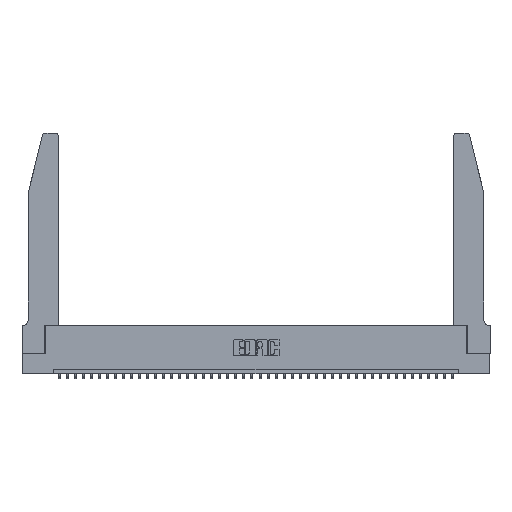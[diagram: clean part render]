
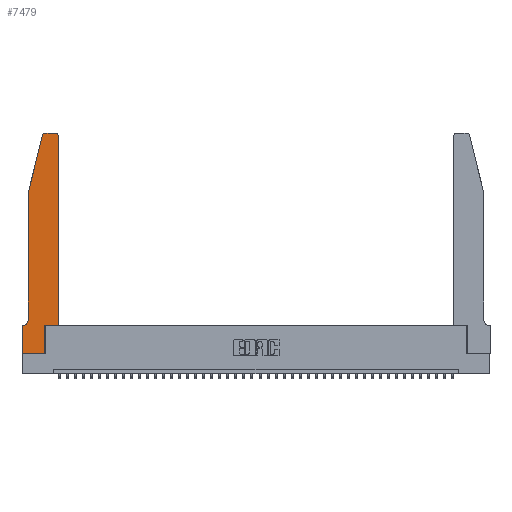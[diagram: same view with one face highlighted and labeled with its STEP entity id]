
A CAD part, top view. The second image highlights one B-rep face of the part: STEP entity #7479.
In plain terms, the highlighted planar face has unit normal (0, 0, 1).
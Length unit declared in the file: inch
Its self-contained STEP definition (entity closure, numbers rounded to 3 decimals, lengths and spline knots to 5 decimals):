
#445 = CIRCLE ( 'NONE', #5407, 0.07 ) ;
#660 = ORIENTED_EDGE ( 'NONE', *, *, #36651, .T. ) ;
#980 = LINE ( 'NONE', #1100, #13918 ) ;
#1089 = DIRECTION ( 'NONE',  ( 0., 1., 0. ) ) ;
#1100 = CARTESIAN_POINT ( 'NONE',  ( 0.0755, 0.35, 0.37 ) ) ;
#1144 = LINE ( 'NONE', #20333, #39673 ) ;
#2079 = VERTEX_POINT ( 'NONE', #34887 ) ;
#2639 = CARTESIAN_POINT ( 'NONE',  ( 0.0055, 0.42, 0.37 ) ) ;
#2670 = AXIS2_PLACEMENT_3D ( 'NONE', #26265, #9977, #19232 ) ;
#2970 = CARTESIAN_POINT ( 'NONE',  ( 0.2605, 2.75, 0.37 ) ) ;
#3090 = DIRECTION ( 'NONE',  ( -1., 0., 0. ) ) ;
#3388 = EDGE_CURVE ( 'NONE', #22989, #13315, #30884, .T. ) ;
#3605 = CARTESIAN_POINT ( 'NONE',  ( 0., 0.35, 0.37 ) ) ;
#3662 = VERTEX_POINT ( 'NONE', #29640 ) ;
#4069 = EDGE_CURVE ( 'NONE', #26466, #6717, #26324, .T. ) ;
#4239 = ORIENTED_EDGE ( 'NONE', *, *, #11849, .T. ) ;
#4356 = ORIENTED_EDGE ( 'NONE', *, *, #33721, .T. ) ;
#5329 = EDGE_CURVE ( 'NONE', #25042, #22989, #18939, .T. ) ;
#5407 = AXIS2_PLACEMENT_3D ( 'NONE', #2639, #41058, #41185 ) ;
#5956 = DIRECTION ( 'NONE',  ( 0., -1., 0. ) ) ;
#6717 = VERTEX_POINT ( 'NONE', #18554 ) ;
#6720 = CARTESIAN_POINT ( 'NONE',  ( 0.4205, 2.72, 0.37 ) ) ;
#6984 = DIRECTION ( 'NONE',  ( 1., 0., 0. ) ) ;
#7212 = LINE ( 'NONE', #34883, #24792 ) ;
#7479 = ADVANCED_FACE ( 'NONE', ( #13696 ), #15965, .T. ) ;
#7750 = VECTOR ( 'NONE', #23394, 39.37008 ) ;
#8639 = CARTESIAN_POINT ( 'NONE',  ( 0.2865, 0.35, 0.37 ) ) ;
#9977 = DIRECTION ( 'NONE',  ( 0., 0., 1. ) ) ;
#10362 = VECTOR ( 'NONE', #11907, 39.37008 ) ;
#10654 = CARTESIAN_POINT ( 'NONE',  ( 0.4505, 0.35, 0.37 ) ) ;
#10797 = VERTEX_POINT ( 'NONE', #8639 ) ;
#10882 = ORIENTED_EDGE ( 'NONE', *, *, #29481, .T. ) ;
#11099 = ORIENTED_EDGE ( 'NONE', *, *, #30509, .T. ) ;
#11497 = CARTESIAN_POINT ( 'NONE',  ( 0., 0., 0.37 ) ) ;
#11849 = EDGE_CURVE ( 'NONE', #6717, #3662, #20352, .T. ) ;
#11907 = DIRECTION ( 'NONE',  ( 0., -1., 0. ) ) ;
#12045 = ORIENTED_EDGE ( 'NONE', *, *, #14701, .T. ) ;
#12327 = ORIENTED_EDGE ( 'NONE', *, *, #28167, .T. ) ;
#12408 = DIRECTION ( 'NONE',  ( -0.239, -0.971, 0. ) ) ;
#12767 = CARTESIAN_POINT ( 'NONE',  ( 0.0055, 0.35, 0.37 ) ) ;
#12967 = DIRECTION ( 'NONE',  ( 0., 0., 1. ) ) ;
#12972 = DIRECTION ( 'NONE',  ( 1., 0., 0. ) ) ;
#13315 = VERTEX_POINT ( 'NONE', #39771 ) ;
#13356 = VERTEX_POINT ( 'NONE', #14232 ) ;
#13696 = FACE_OUTER_BOUND ( 'NONE', #23552, .T. ) ;
#13918 = VECTOR ( 'NONE', #17854, 39.37008 ) ;
#14232 = CARTESIAN_POINT ( 'NONE',  ( 0.284, 2.75, 0.37 ) ) ;
#14701 = EDGE_CURVE ( 'NONE', #13315, #10797, #1144, .T. ) ;
#14838 = ORIENTED_EDGE ( 'NONE', *, *, #5329, .T. ) ;
#15355 = LINE ( 'NONE', #22701, #17322 ) ;
#15965 = PLANE ( 'NONE',  #31939 ) ;
#16885 = EDGE_CURVE ( 'NONE', #30762, #25042, #980, .T. ) ;
#17322 = VECTOR ( 'NONE', #19857, 39.37008 ) ;
#17854 = DIRECTION ( 'NONE',  ( -1., 0., 0. ) ) ;
#18039 = LINE ( 'NONE', #31436, #19452 ) ;
#18554 = CARTESIAN_POINT ( 'NONE',  ( 0.4505, 2.72, 0.37 ) ) ;
#18585 = CARTESIAN_POINT ( 'NONE',  ( 0., 0., 0.37 ) ) ;
#18750 = CIRCLE ( 'NONE', #2670, 0.03 ) ;
#18935 = EDGE_CURVE ( 'NONE', #2079, #21942, #7212, .T. ) ;
#18939 = LINE ( 'NONE', #11497, #10362 ) ;
#19153 = CARTESIAN_POINT ( 'NONE',  ( 0.0755, 0.42, 0.37 ) ) ;
#19232 = DIRECTION ( 'NONE',  ( 1., 0., 0. ) ) ;
#19293 = CARTESIAN_POINT ( 'NONE',  ( 0., 0.35, 0.37 ) ) ;
#19452 = VECTOR ( 'NONE', #5956, 39.37008 ) ;
#19857 = DIRECTION ( 'NONE',  ( 1., 0., 0. ) ) ;
#20333 = CARTESIAN_POINT ( 'NONE',  ( 0.2865, 0.35, 0.37 ) ) ;
#20352 = CIRCLE ( 'NONE', #22343, 0.03 ) ;
#21487 = ORIENTED_EDGE ( 'NONE', *, *, #16885, .T. ) ;
#21905 = VECTOR ( 'NONE', #12972, 39.37008 ) ;
#21942 = VERTEX_POINT ( 'NONE', #40356 ) ;
#22343 = AXIS2_PLACEMENT_3D ( 'NONE', #6720, #12967, #29147 ) ;
#22701 = CARTESIAN_POINT ( 'NONE',  ( 0.4505, 0.35, 0.37 ) ) ;
#22989 = VERTEX_POINT ( 'NONE', #29542 ) ;
#23394 = DIRECTION ( 'NONE',  ( 0., 1., 0. ) ) ;
#23552 = EDGE_LOOP ( 'NONE', ( #11099, #660, #39638, #4356, #12327, #21487, #14838, #31108, #12045, #10882, #35441, #4239 ) ) ;
#23817 = LINE ( 'NONE', #2970, #27361 ) ;
#24792 = VECTOR ( 'NONE', #12408, 39.37008 ) ;
#25042 = VERTEX_POINT ( 'NONE', #3605 ) ;
#26265 = CARTESIAN_POINT ( 'NONE',  ( 0.284, 2.72, 0.37 ) ) ;
#26324 = LINE ( 'NONE', #36262, #7750 ) ;
#26466 = VERTEX_POINT ( 'NONE', #10654 ) ;
#27361 = VECTOR ( 'NONE', #3090, 39.37008 ) ;
#28167 = EDGE_CURVE ( 'NONE', #31678, #30762, #445, .T. ) ;
#29147 = DIRECTION ( 'NONE',  ( 1., 0., 0. ) ) ;
#29481 = EDGE_CURVE ( 'NONE', #10797, #26466, #15355, .T. ) ;
#29542 = CARTESIAN_POINT ( 'NONE',  ( 0., 0., 0.37 ) ) ;
#29640 = CARTESIAN_POINT ( 'NONE',  ( 0.4205, 2.75, 0.37 ) ) ;
#30509 = EDGE_CURVE ( 'NONE', #3662, #13356, #23817, .T. ) ;
#30762 = VERTEX_POINT ( 'NONE', #12767 ) ;
#30884 = LINE ( 'NONE', #18585, #21905 ) ;
#31108 = ORIENTED_EDGE ( 'NONE', *, *, #3388, .T. ) ;
#31436 = CARTESIAN_POINT ( 'NONE',  ( 0.0755, 2., 0.37 ) ) ;
#31678 = VERTEX_POINT ( 'NONE', #19153 ) ;
#31939 = AXIS2_PLACEMENT_3D ( 'NONE', #19293, #32457, #6984 ) ;
#32457 = DIRECTION ( 'NONE',  ( 0., 0., 1. ) ) ;
#33721 = EDGE_CURVE ( 'NONE', #21942, #31678, #18039, .T. ) ;
#34883 = CARTESIAN_POINT ( 'NONE',  ( 0.0755, 2., 0.37 ) ) ;
#34887 = CARTESIAN_POINT ( 'NONE',  ( 0.25487, 2.72718, 0.37 ) ) ;
#35441 = ORIENTED_EDGE ( 'NONE', *, *, #4069, .T. ) ;
#36262 = CARTESIAN_POINT ( 'NONE',  ( 0.4505, 0.35, 0.37 ) ) ;
#36651 = EDGE_CURVE ( 'NONE', #13356, #2079, #18750, .T. ) ;
#39638 = ORIENTED_EDGE ( 'NONE', *, *, #18935, .T. ) ;
#39673 = VECTOR ( 'NONE', #1089, 39.37008 ) ;
#39771 = CARTESIAN_POINT ( 'NONE',  ( 0.2865, 0., 0.37 ) ) ;
#40356 = CARTESIAN_POINT ( 'NONE',  ( 0.0755, 2., 0.37 ) ) ;
#41058 = DIRECTION ( 'NONE',  ( 0., 0., -1. ) ) ;
#41185 = DIRECTION ( 'NONE',  ( -1., 0., 0. ) ) ;
